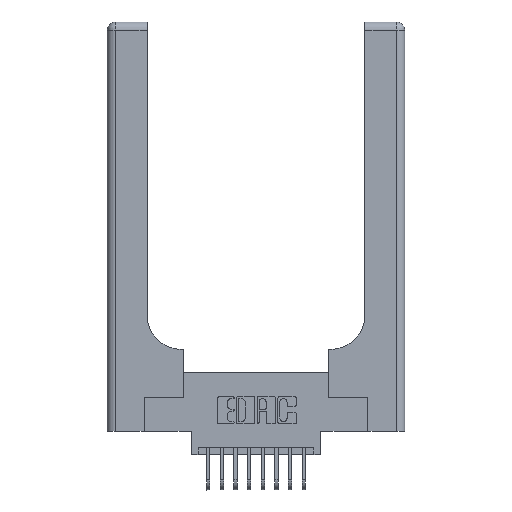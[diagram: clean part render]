
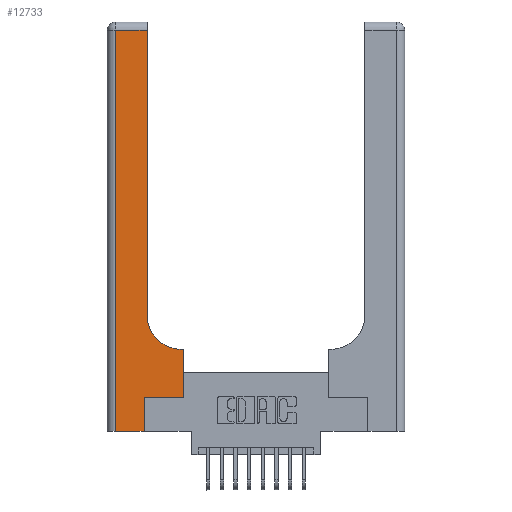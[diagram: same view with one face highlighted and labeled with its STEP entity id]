
A CAD part, top view. The second image highlights one B-rep face of the part: STEP entity #12733.
In plain terms, the highlighted planar face has unit normal (0, 0, 1).
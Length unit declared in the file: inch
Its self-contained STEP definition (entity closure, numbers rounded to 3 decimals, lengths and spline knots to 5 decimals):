
#166 = EDGE_LOOP ( 'NONE', ( #11507, #10085, #3696, #1273, #12246, #3202, #7826, #5619, #12907 ) ) ;
#568 = LINE ( 'NONE', #3057, #8250 ) ;
#751 = VECTOR ( 'NONE', #7998, 39.37008 ) ;
#823 = EDGE_CURVE ( 'NONE', #6686, #6612, #14168, .T. ) ;
#956 = EDGE_CURVE ( 'NONE', #2940, #11708, #2703, .T. ) ;
#1254 = CARTESIAN_POINT ( 'NONE',  ( 0.269, 0.25, 0.37 ) ) ;
#1273 = ORIENTED_EDGE ( 'NONE', *, *, #13864, .T. ) ;
#1445 = CARTESIAN_POINT ( 'NONE',  ( 0.269, 0., 0.37 ) ) ;
#1504 = EDGE_CURVE ( 'NONE', #11708, #3601, #10762, .T. ) ;
#2703 = LINE ( 'NONE', #12845, #9301 ) ;
#2940 = VERTEX_POINT ( 'NONE', #12632 ) ;
#3021 = EDGE_CURVE ( 'NONE', #3601, #13870, #11786, .T. ) ;
#3057 = CARTESIAN_POINT ( 'NONE',  ( 0.06, 3., 0.37 ) ) ;
#3199 = CARTESIAN_POINT ( 'NONE',  ( 0., 3., 0.37 ) ) ;
#3202 = ORIENTED_EDGE ( 'NONE', *, *, #823, .T. ) ;
#3513 = VERTEX_POINT ( 'NONE', #13566 ) ;
#3601 = VERTEX_POINT ( 'NONE', #10278 ) ;
#3696 = ORIENTED_EDGE ( 'NONE', *, *, #6566, .T. ) ;
#4132 = DIRECTION ( 'NONE',  ( 0., 1., 0. ) ) ;
#4251 = DIRECTION ( 'NONE',  ( 0., 1., 0. ) ) ;
#4519 = DIRECTION ( 'NONE',  ( 0., -1., 0. ) ) ;
#4658 = PLANE ( 'NONE',  #12671 ) ;
#4678 = EDGE_CURVE ( 'NONE', #6612, #2940, #8488, .T. ) ;
#5619 = ORIENTED_EDGE ( 'NONE', *, *, #956, .T. ) ;
#6007 = DIRECTION ( 'NONE',  ( -1., 0., 0. ) ) ;
#6074 = VECTOR ( 'NONE', #4251, 39.37008 ) ;
#6454 = CARTESIAN_POINT ( 'NONE',  ( 0., 2.94, 0.37 ) ) ;
#6462 = EDGE_CURVE ( 'NONE', #14615, #6686, #15353, .T. ) ;
#6524 = DIRECTION ( 'NONE',  ( 0., 0., -1. ) ) ;
#6555 = VERTEX_POINT ( 'NONE', #10697 ) ;
#6566 = EDGE_CURVE ( 'NONE', #3513, #6555, #568, .T. ) ;
#6612 = VERTEX_POINT ( 'NONE', #14236 ) ;
#6686 = VERTEX_POINT ( 'NONE', #10897 ) ;
#6944 = DIRECTION ( 'NONE',  ( -1., 0., 0. ) ) ;
#7449 = CARTESIAN_POINT ( 'NONE',  ( 0.269, 0., 0.37 ) ) ;
#7600 = AXIS2_PLACEMENT_3D ( 'NONE', #13654, #6524, #14721 ) ;
#7774 = DIRECTION ( 'NONE',  ( 1., 0., 0. ) ) ;
#7826 = ORIENTED_EDGE ( 'NONE', *, *, #4678, .T. ) ;
#7998 = DIRECTION ( 'NONE',  ( 1., 0., 0. ) ) ;
#8250 = VECTOR ( 'NONE', #4519, 39.37008 ) ;
#8482 = VECTOR ( 'NONE', #13589, 39.37008 ) ;
#8488 = LINE ( 'NONE', #9775, #11554 ) ;
#9024 = CARTESIAN_POINT ( 'NONE',  ( 0.2915, 2.94, 0.37 ) ) ;
#9301 = VECTOR ( 'NONE', #6944, 39.37008 ) ;
#9670 = DIRECTION ( 'NONE',  ( 0., 0., -1. ) ) ;
#9775 = CARTESIAN_POINT ( 'NONE',  ( 0.5585, 0.25, 0.37 ) ) ;
#10085 = ORIENTED_EDGE ( 'NONE', *, *, #11407, .T. ) ;
#10278 = CARTESIAN_POINT ( 'NONE',  ( 0.2915, 0.85, 0.37 ) ) ;
#10697 = CARTESIAN_POINT ( 'NONE',  ( 0.06, 0., 0.37 ) ) ;
#10762 = CIRCLE ( 'NONE', #7600, 0.25 ) ;
#10897 = CARTESIAN_POINT ( 'NONE',  ( 0.269, 0.25, 0.37 ) ) ;
#11407 = EDGE_CURVE ( 'NONE', #13870, #3513, #12269, .T. ) ;
#11424 = VECTOR ( 'NONE', #4132, 39.37008 ) ;
#11507 = ORIENTED_EDGE ( 'NONE', *, *, #3021, .T. ) ;
#11554 = VECTOR ( 'NONE', #13280, 39.37008 ) ;
#11587 = CARTESIAN_POINT ( 'NONE',  ( 0.2915, 3., 0.37 ) ) ;
#11708 = VERTEX_POINT ( 'NONE', #14366 ) ;
#11786 = LINE ( 'NONE', #11587, #11424 ) ;
#12246 = ORIENTED_EDGE ( 'NONE', *, *, #6462, .T. ) ;
#12269 = LINE ( 'NONE', #6454, #8482 ) ;
#12425 = CARTESIAN_POINT ( 'NONE',  ( 0., 0., 0.37 ) ) ;
#12632 = CARTESIAN_POINT ( 'NONE',  ( 0.5585, 0.6, 0.37 ) ) ;
#12671 = AXIS2_PLACEMENT_3D ( 'NONE', #3199, #9670, #6007 ) ;
#12733 = ADVANCED_FACE ( 'NONE', ( #14568 ), #4658, .F. ) ;
#12845 = CARTESIAN_POINT ( 'NONE',  ( 0.2915, 0.6, 0.37 ) ) ;
#12907 = ORIENTED_EDGE ( 'NONE', *, *, #1504, .T. ) ;
#13185 = VECTOR ( 'NONE', #7774, 39.37008 ) ;
#13280 = DIRECTION ( 'NONE',  ( 0., 1., 0. ) ) ;
#13566 = CARTESIAN_POINT ( 'NONE',  ( 0.06, 2.94, 0.37 ) ) ;
#13589 = DIRECTION ( 'NONE',  ( -1., 0., 0. ) ) ;
#13654 = CARTESIAN_POINT ( 'NONE',  ( 0.5415, 0.85, 0.37 ) ) ;
#13864 = EDGE_CURVE ( 'NONE', #6555, #14615, #15953, .T. ) ;
#13870 = VERTEX_POINT ( 'NONE', #9024 ) ;
#14168 = LINE ( 'NONE', #1254, #751 ) ;
#14236 = CARTESIAN_POINT ( 'NONE',  ( 0.5585, 0.25, 0.37 ) ) ;
#14366 = CARTESIAN_POINT ( 'NONE',  ( 0.5415, 0.6, 0.37 ) ) ;
#14568 = FACE_OUTER_BOUND ( 'NONE', #166, .T. ) ;
#14615 = VERTEX_POINT ( 'NONE', #7449 ) ;
#14721 = DIRECTION ( 'NONE',  ( 1., 0., 0. ) ) ;
#15353 = LINE ( 'NONE', #1445, #6074 ) ;
#15953 = LINE ( 'NONE', #12425, #13185 ) ;
